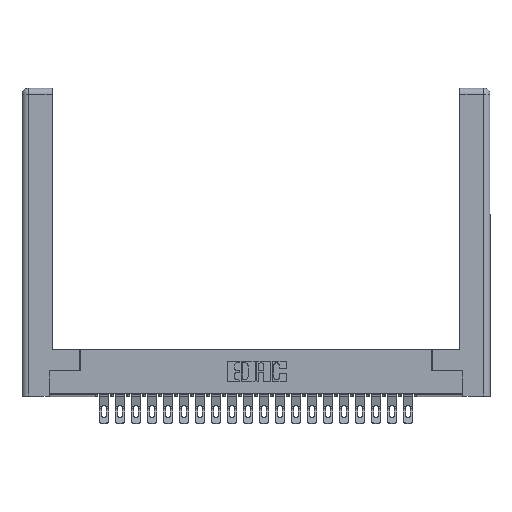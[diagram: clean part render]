
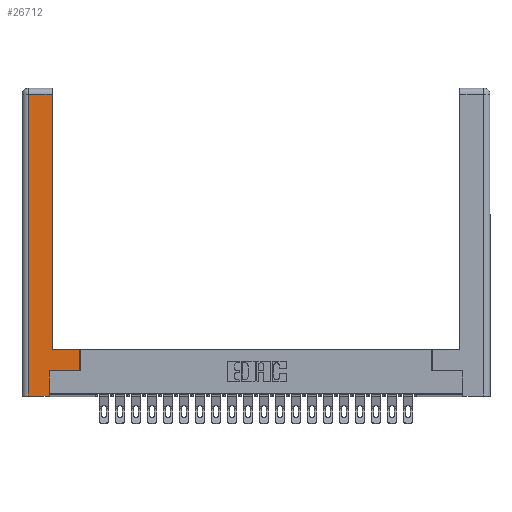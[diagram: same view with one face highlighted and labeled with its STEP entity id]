
A CAD part, top view. The second image highlights one B-rep face of the part: STEP entity #26712.
In plain terms, the highlighted planar face has unit normal (0, 0, 1).
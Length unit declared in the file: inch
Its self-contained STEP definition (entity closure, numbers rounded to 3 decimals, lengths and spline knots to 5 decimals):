
#241 = LINE ( 'NONE', #6048, #16873 ) ;
#530 = CARTESIAN_POINT ( 'NONE',  ( 0.295, 3., 0. ) ) ;
#1306 = VERTEX_POINT ( 'NONE', #5933 ) ;
#1504 = ORIENTED_EDGE ( 'NONE', *, *, #17323, .T. ) ;
#1506 = DIRECTION ( 'NONE',  ( 0., 0., -1. ) ) ;
#1745 = VECTOR ( 'NONE', #26597, 39.37008 ) ;
#1991 = EDGE_CURVE ( 'NONE', #5919, #24993, #13390, .T. ) ;
#3012 = PLANE ( 'NONE',  #16754 ) ;
#3230 = ORIENTED_EDGE ( 'NONE', *, *, #1991, .T. ) ;
#3315 = CARTESIAN_POINT ( 'NONE',  ( 0.565, 0.45, 0. ) ) ;
#3750 = DIRECTION ( 'NONE',  ( -1., 0., 0. ) ) ;
#4359 = CARTESIAN_POINT ( 'NONE',  ( 0.0615, 2.94, 0. ) ) ;
#5001 = CARTESIAN_POINT ( 'NONE',  ( 0.295, 2.94, 0. ) ) ;
#5044 = CARTESIAN_POINT ( 'NONE',  ( 0.295, 0.45, 0. ) ) ;
#5471 = DIRECTION ( 'NONE',  ( 0., 1., 0. ) ) ;
#5542 = EDGE_CURVE ( 'NONE', #1306, #24245, #241, .T. ) ;
#5919 = VERTEX_POINT ( 'NONE', #5001 ) ;
#5933 = CARTESIAN_POINT ( 'NONE',  ( 0.565, 0.45, 0. ) ) ;
#6048 = CARTESIAN_POINT ( 'NONE',  ( 0.295, 0.45, 0. ) ) ;
#6405 = DIRECTION ( 'NONE',  ( -1., 0., 0. ) ) ;
#6418 = ORIENTED_EDGE ( 'NONE', *, *, #17919, .T. ) ;
#6738 = CARTESIAN_POINT ( 'NONE',  ( 0.565, 0.245, 0. ) ) ;
#7255 = EDGE_CURVE ( 'NONE', #24993, #17362, #12226, .T. ) ;
#7595 = VECTOR ( 'NONE', #5471, 39.37008 ) ;
#8514 = EDGE_LOOP ( 'NONE', ( #1504, #3230, #24090, #21781, #6418, #20764, #20318, #23510 ) ) ;
#9593 = VECTOR ( 'NONE', #21952, 39.37008 ) ;
#9846 = DIRECTION ( 'NONE',  ( 1., 0., 0. ) ) ;
#12226 = LINE ( 'NONE', #20894, #17242 ) ;
#12278 = CARTESIAN_POINT ( 'NONE',  ( 0.0615, 2.94, 0. ) ) ;
#12311 = EDGE_CURVE ( 'NONE', #21170, #1306, #14253, .T. ) ;
#13352 = FACE_OUTER_BOUND ( 'NONE', #8514, .T. ) ;
#13390 = LINE ( 'NONE', #4359, #21738 ) ;
#13892 = VECTOR ( 'NONE', #26025, 39.37008 ) ;
#14253 = LINE ( 'NONE', #3315, #7595 ) ;
#14737 = LINE ( 'NONE', #16332, #1745 ) ;
#15444 = VERTEX_POINT ( 'NONE', #18296 ) ;
#15595 = CARTESIAN_POINT ( 'NONE',  ( 0.0615, 0., 0. ) ) ;
#15858 = VERTEX_POINT ( 'NONE', #20048 ) ;
#16332 = CARTESIAN_POINT ( 'NONE',  ( 0.565, 0.245, 0. ) ) ;
#16569 = LINE ( 'NONE', #21637, #13892 ) ;
#16754 = AXIS2_PLACEMENT_3D ( 'NONE', #19856, #1506, #3750 ) ;
#16873 = VECTOR ( 'NONE', #6405, 39.37008 ) ;
#16974 = DIRECTION ( 'NONE',  ( 0., -1., 0. ) ) ;
#17242 = VECTOR ( 'NONE', #16974, 39.37008 ) ;
#17323 = EDGE_CURVE ( 'NONE', #24245, #5919, #25280, .T. ) ;
#17362 = VERTEX_POINT ( 'NONE', #15595 ) ;
#17919 = EDGE_CURVE ( 'NONE', #15858, #15444, #16569, .T. ) ;
#17981 = VECTOR ( 'NONE', #9846, 39.37008 ) ;
#18296 = CARTESIAN_POINT ( 'NONE',  ( 0.265, 0.245, 0. ) ) ;
#19236 = DIRECTION ( 'NONE',  ( -1., 0., 0. ) ) ;
#19856 = CARTESIAN_POINT ( 'NONE',  ( 0., 0., 0. ) ) ;
#20048 = CARTESIAN_POINT ( 'NONE',  ( 0.265, 0., 0. ) ) ;
#20318 = ORIENTED_EDGE ( 'NONE', *, *, #12311, .T. ) ;
#20764 = ORIENTED_EDGE ( 'NONE', *, *, #20873, .T. ) ;
#20873 = EDGE_CURVE ( 'NONE', #15444, #21170, #14737, .T. ) ;
#20894 = CARTESIAN_POINT ( 'NONE',  ( 0.0615, 0., 0. ) ) ;
#21170 = VERTEX_POINT ( 'NONE', #6738 ) ;
#21637 = CARTESIAN_POINT ( 'NONE',  ( 0.265, 0.245, 0. ) ) ;
#21738 = VECTOR ( 'NONE', #19236, 39.37008 ) ;
#21781 = ORIENTED_EDGE ( 'NONE', *, *, #22102, .T. ) ;
#21952 = DIRECTION ( 'NONE',  ( 0., 1., 0. ) ) ;
#22102 = EDGE_CURVE ( 'NONE', #17362, #15858, #23657, .T. ) ;
#23510 = ORIENTED_EDGE ( 'NONE', *, *, #5542, .T. ) ;
#23657 = LINE ( 'NONE', #24860, #17981 ) ;
#24090 = ORIENTED_EDGE ( 'NONE', *, *, #7255, .T. ) ;
#24245 = VERTEX_POINT ( 'NONE', #5044 ) ;
#24860 = CARTESIAN_POINT ( 'NONE',  ( 0.265, 0., 0. ) ) ;
#24993 = VERTEX_POINT ( 'NONE', #12278 ) ;
#25280 = LINE ( 'NONE', #530, #9593 ) ;
#26025 = DIRECTION ( 'NONE',  ( 0., 1., 0. ) ) ;
#26597 = DIRECTION ( 'NONE',  ( 1., 0., 0. ) ) ;
#26712 = ADVANCED_FACE ( 'NONE', ( #13352 ), #3012, .F. ) ;
